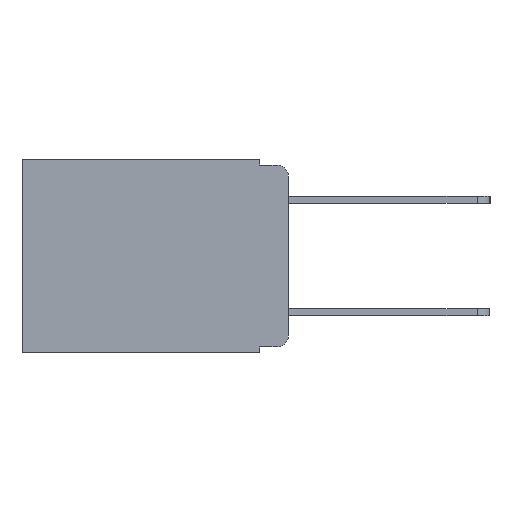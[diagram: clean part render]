
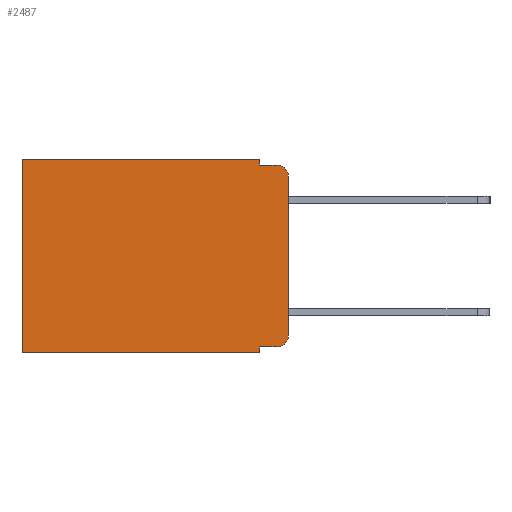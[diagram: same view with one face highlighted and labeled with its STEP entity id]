
A CAD part, left-side view. The second image highlights one B-rep face of the part: STEP entity #2487.
In plain terms, the highlighted planar face has unit normal (-1, 0, 0).
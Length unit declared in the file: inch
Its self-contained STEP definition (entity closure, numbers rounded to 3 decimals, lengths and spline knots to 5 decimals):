
#201 = EDGE_CURVE ( 'NONE', #5456, #12852, #3020, .T. ) ;
#327 = CARTESIAN_POINT ( 'NONE',  ( 0.298, 0.051, 0. ) ) ;
#385 = EDGE_CURVE ( 'NONE', #5346, #12852, #8697, .T. ) ;
#479 = EDGE_CURVE ( 'NONE', #12252, #5346, #6380, .T. ) ;
#547 = CARTESIAN_POINT ( 'NONE',  ( 0.298, 0., 0. ) ) ;
#560 = DIRECTION ( 'NONE',  ( 0., -1., 0. ) ) ;
#625 = VERTEX_POINT ( 'NONE', #10844 ) ;
#631 = EDGE_CURVE ( 'NONE', #625, #6075, #13993, .T. ) ;
#692 = EDGE_CURVE ( 'NONE', #4505, #13435, #12676, .T. ) ;
#730 = EDGE_CURVE ( 'NONE', #4505, #4850, #15152, .T. ) ;
#831 = EDGE_CURVE ( 'NONE', #4850, #13727, #13815, .T. ) ;
#1067 = LINE ( 'NONE', #547, #7197 ) ;
#1741 = AXIS2_PLACEMENT_3D ( 'NONE', #7565, #8872, #7368 ) ;
#1786 = CARTESIAN_POINT ( 'NONE',  ( 0.298, 0.051, -0.343 ) ) ;
#2035 = DIRECTION ( 'NONE',  ( 0., 0., -1. ) ) ;
#2087 = DIRECTION ( 'NONE',  ( 0., 1., 0. ) ) ;
#2487 = ADVANCED_FACE ( 'NONE', ( #14923 ), #8875, .F. ) ;
#2838 = VECTOR ( 'NONE', #9787, 39.37008 ) ;
#2856 = VECTOR ( 'NONE', #12904, 39.37008 ) ;
#2863 = CARTESIAN_POINT ( 'NONE',  ( 0.298, 0.02, -0.313 ) ) ;
#2960 = VECTOR ( 'NONE', #2087, 39.37008 ) ;
#3020 = CIRCLE ( 'NONE', #1741, 0.02 ) ;
#3358 = EDGE_LOOP ( 'NONE', ( #11110, #7771, #8376, #7312, #8719, #7930, #9410, #8391, #9422, #9113 ) ) ;
#3555 = CARTESIAN_POINT ( 'NONE',  ( 0.298, 0.051, -0.01 ) ) ;
#3872 = CARTESIAN_POINT ( 'NONE',  ( 0.298, 0.051, -0.333 ) ) ;
#4210 = DIRECTION ( 'NONE',  ( 0., 0., -1. ) ) ;
#4505 = VERTEX_POINT ( 'NONE', #3872 ) ;
#4850 = VERTEX_POINT ( 'NONE', #9350 ) ;
#5074 = VECTOR ( 'NONE', #9001, 39.37008 ) ;
#5346 = VERTEX_POINT ( 'NONE', #10428 ) ;
#5412 = LINE ( 'NONE', #7848, #5074 ) ;
#5456 = VERTEX_POINT ( 'NONE', #9058 ) ;
#5741 = CARTESIAN_POINT ( 'NONE',  ( 0.298, 0., -0.343 ) ) ;
#6075 = VERTEX_POINT ( 'NONE', #11409 ) ;
#6120 = LINE ( 'NONE', #5741, #2960 ) ;
#6209 = CARTESIAN_POINT ( 'NONE',  ( 0.298, 0.473, 0. ) ) ;
#6259 = CARTESIAN_POINT ( 'NONE',  ( 0.298, 0.051, -0.333 ) ) ;
#6278 = CARTESIAN_POINT ( 'NONE',  ( 0.298, 0.051, 0. ) ) ;
#6380 = LINE ( 'NONE', #327, #2856 ) ;
#6726 = AXIS2_PLACEMENT_3D ( 'NONE', #7554, #9127, #2035 ) ;
#6742 = DIRECTION ( 'NONE',  ( 0., 0., -1. ) ) ;
#7081 = CARTESIAN_POINT ( 'NONE',  ( 0.298, 0.02, -0.01 ) ) ;
#7197 = VECTOR ( 'NONE', #9322, 39.37008 ) ;
#7312 = ORIENTED_EDGE ( 'NONE', *, *, #479, .F. ) ;
#7368 = DIRECTION ( 'NONE',  ( 0., 0., -1. ) ) ;
#7554 = CARTESIAN_POINT ( 'NONE',  ( 0.298, 0., 0. ) ) ;
#7565 = CARTESIAN_POINT ( 'NONE',  ( 0.298, 0.02, -0.03 ) ) ;
#7771 = ORIENTED_EDGE ( 'NONE', *, *, #201, .T. ) ;
#7848 = CARTESIAN_POINT ( 'NONE',  ( 0.298, 0., 0. ) ) ;
#7930 = ORIENTED_EDGE ( 'NONE', *, *, #631, .T. ) ;
#8128 = DIRECTION ( 'NONE',  ( 0., 0., -1. ) ) ;
#8376 = ORIENTED_EDGE ( 'NONE', *, *, #385, .F. ) ;
#8391 = ORIENTED_EDGE ( 'NONE', *, *, #692, .F. ) ;
#8697 = LINE ( 'NONE', #3555, #11298 ) ;
#8719 = ORIENTED_EDGE ( 'NONE', *, *, #12312, .T. ) ;
#8872 = DIRECTION ( 'NONE',  ( -1., 0., 0. ) ) ;
#8875 = PLANE ( 'NONE',  #6726 ) ;
#9001 = DIRECTION ( 'NONE',  ( 0., 0., -1. ) ) ;
#9058 = CARTESIAN_POINT ( 'NONE',  ( 0.298, 0., -0.03 ) ) ;
#9113 = ORIENTED_EDGE ( 'NONE', *, *, #831, .T. ) ;
#9127 = DIRECTION ( 'NONE',  ( 1., 0., 0. ) ) ;
#9322 = DIRECTION ( 'NONE',  ( 0., 1., 0. ) ) ;
#9350 = CARTESIAN_POINT ( 'NONE',  ( 0.298, 0.02, -0.333 ) ) ;
#9410 = ORIENTED_EDGE ( 'NONE', *, *, #14113, .F. ) ;
#9422 = ORIENTED_EDGE ( 'NONE', *, *, #730, .T. ) ;
#9717 = VECTOR ( 'NONE', #8128, 39.37008 ) ;
#9787 = DIRECTION ( 'NONE',  ( 0., -1., 0. ) ) ;
#10428 = CARTESIAN_POINT ( 'NONE',  ( 0.298, 0.051, -0.01 ) ) ;
#10844 = CARTESIAN_POINT ( 'NONE',  ( 0.298, 0.473, 0. ) ) ;
#10888 = CARTESIAN_POINT ( 'NONE',  ( 0.298, 0.051, 0. ) ) ;
#11110 = ORIENTED_EDGE ( 'NONE', *, *, #14629, .F. ) ;
#11140 = VECTOR ( 'NONE', #6742, 39.37008 ) ;
#11298 = VECTOR ( 'NONE', #560, 39.37008 ) ;
#11409 = CARTESIAN_POINT ( 'NONE',  ( 0.298, 0.473, -0.343 ) ) ;
#12252 = VERTEX_POINT ( 'NONE', #10888 ) ;
#12312 = EDGE_CURVE ( 'NONE', #12252, #625, #1067, .T. ) ;
#12456 = AXIS2_PLACEMENT_3D ( 'NONE', #2863, #13721, #4210 ) ;
#12511 = CARTESIAN_POINT ( 'NONE',  ( 0.298, 0., -0.313 ) ) ;
#12676 = LINE ( 'NONE', #6278, #9717 ) ;
#12852 = VERTEX_POINT ( 'NONE', #7081 ) ;
#12904 = DIRECTION ( 'NONE',  ( 0., 0., -1. ) ) ;
#13435 = VERTEX_POINT ( 'NONE', #1786 ) ;
#13721 = DIRECTION ( 'NONE',  ( -1., 0., 0. ) ) ;
#13727 = VERTEX_POINT ( 'NONE', #12511 ) ;
#13815 = CIRCLE ( 'NONE', #12456, 0.02 ) ;
#13993 = LINE ( 'NONE', #6209, #11140 ) ;
#14113 = EDGE_CURVE ( 'NONE', #13435, #6075, #6120, .T. ) ;
#14629 = EDGE_CURVE ( 'NONE', #5456, #13727, #5412, .T. ) ;
#14923 = FACE_OUTER_BOUND ( 'NONE', #3358, .T. ) ;
#15152 = LINE ( 'NONE', #6259, #2838 ) ;
